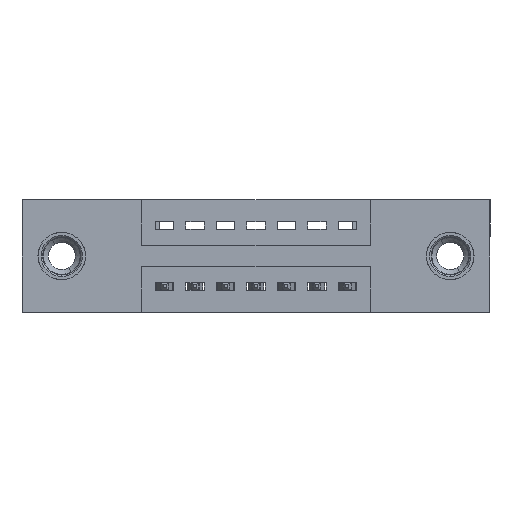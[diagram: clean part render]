
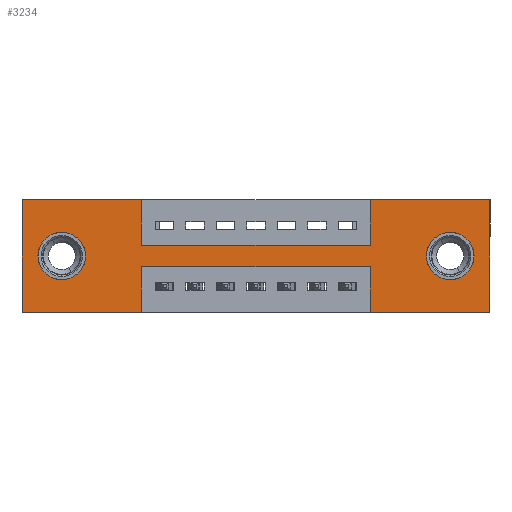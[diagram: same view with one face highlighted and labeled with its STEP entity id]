
A CAD part, front view. The second image highlights one B-rep face of the part: STEP entity #3234.
In plain terms, the highlighted planar face has unit normal (0, -1, 0).
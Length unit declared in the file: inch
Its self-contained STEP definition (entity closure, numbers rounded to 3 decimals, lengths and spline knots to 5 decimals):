
#51 = LINE ( 'NONE', #2546, #246 ) ;
#246 = VECTOR ( 'NONE', #10534, 39.37008 ) ;
#383 = DIRECTION ( 'NONE',  ( 0., -1., 0. ) ) ;
#586 = VERTEX_POINT ( 'NONE', #7537 ) ;
#606 = VERTEX_POINT ( 'NONE', #13101 ) ;
#614 = VERTEX_POINT ( 'NONE', #13140 ) ;
#677 = EDGE_LOOP ( 'NONE', ( #12969, #3364 ) ) ;
#689 = VECTOR ( 'NONE', #7969, 39.37008 ) ;
#757 = ORIENTED_EDGE ( 'NONE', *, *, #4747, .F. ) ;
#789 = EDGE_CURVE ( 'NONE', #6953, #606, #9669, .T. ) ;
#833 = VERTEX_POINT ( 'NONE', #7582 ) ;
#1064 = EDGE_CURVE ( 'NONE', #606, #586, #51, .T. ) ;
#1142 = EDGE_CURVE ( 'NONE', #3409, #6013, #7853, .T. ) ;
#1166 = LINE ( 'NONE', #12140, #6649 ) ;
#1237 = AXIS2_PLACEMENT_3D ( 'NONE', #4250, #4200, #7701 ) ;
#1314 = DIRECTION ( 'NONE',  ( -1., 0., 0. ) ) ;
#1387 = DIRECTION ( 'NONE',  ( 0., 1., 0. ) ) ;
#1470 = LINE ( 'NONE', #12264, #11460 ) ;
#1764 = ORIENTED_EDGE ( 'NONE', *, *, #7753, .F. ) ;
#1964 = CARTESIAN_POINT ( 'NONE',  ( 0., 0., -0.37 ) ) ;
#2014 = ORIENTED_EDGE ( 'NONE', *, *, #13558, .F. ) ;
#2113 = CARTESIAN_POINT ( 'NONE',  ( 0., 0., 0. ) ) ;
#2198 = CARTESIAN_POINT ( 'NONE',  ( 0.13, 0., -0.185 ) ) ;
#2272 = CARTESIAN_POINT ( 'NONE',  ( 0.3925, 0., 0. ) ) ;
#2278 = FACE_BOUND ( 'NONE', #6630, .T. ) ;
#2400 = EDGE_CURVE ( 'NONE', #7085, #12462, #4074, .T. ) ;
#2546 = CARTESIAN_POINT ( 'NONE',  ( 1.1425, 0., -0.37 ) ) ;
#2766 = CARTESIAN_POINT ( 'NONE',  ( 0.3925, 0., -0.22 ) ) ;
#2775 = ORIENTED_EDGE ( 'NONE', *, *, #1142, .T. ) ;
#2956 = CARTESIAN_POINT ( 'NONE',  ( 0.13, 0., -0.263 ) ) ;
#3073 = CARTESIAN_POINT ( 'NONE',  ( 1.535, 0., 0. ) ) ;
#3091 = DIRECTION ( 'NONE',  ( 0., 0., 1. ) ) ;
#3234 = ADVANCED_FACE ( 'NONE', ( #3869, #2278, #10321 ), #11690, .T. ) ;
#3237 = EDGE_LOOP ( 'NONE', ( #12624, #14509, #9939, #12177, #757, #9696, #1764, #8706, #6977, #9450, #2014, #5295 ) ) ;
#3364 = ORIENTED_EDGE ( 'NONE', *, *, #11262, .T. ) ;
#3375 = LINE ( 'NONE', #12848, #5713 ) ;
#3377 = VERTEX_POINT ( 'NONE', #3429 ) ;
#3391 = CARTESIAN_POINT ( 'NONE',  ( 0.3925, 0., -0.15 ) ) ;
#3409 = VERTEX_POINT ( 'NONE', #14288 ) ;
#3429 = CARTESIAN_POINT ( 'NONE',  ( 1.405, 0., -0.263 ) ) ;
#3604 = LINE ( 'NONE', #7805, #10917 ) ;
#3758 = EDGE_CURVE ( 'NONE', #6013, #3409, #10312, .T. ) ;
#3869 = FACE_BOUND ( 'NONE', #677, .T. ) ;
#4074 = LINE ( 'NONE', #5145, #10182 ) ;
#4200 = DIRECTION ( 'NONE',  ( 0., 1., 0. ) ) ;
#4250 = CARTESIAN_POINT ( 'NONE',  ( 1.405, 0., -0.185 ) ) ;
#4520 = LINE ( 'NONE', #13825, #13256 ) ;
#4596 = DIRECTION ( 'NONE',  ( 0., 0., 1. ) ) ;
#4747 = EDGE_CURVE ( 'NONE', #13995, #6953, #8830, .T. ) ;
#5145 = CARTESIAN_POINT ( 'NONE',  ( 0.3925, 0., -0.37 ) ) ;
#5265 = EDGE_CURVE ( 'NONE', #11827, #3377, #8095, .T. ) ;
#5295 = ORIENTED_EDGE ( 'NONE', *, *, #13341, .F. ) ;
#5491 = DIRECTION ( 'NONE',  ( 0., 0., 1. ) ) ;
#5689 = CARTESIAN_POINT ( 'NONE',  ( 0.3925, 0., -0.37 ) ) ;
#5713 = VECTOR ( 'NONE', #6033, 39.37008 ) ;
#6013 = VERTEX_POINT ( 'NONE', #2956 ) ;
#6033 = DIRECTION ( 'NONE',  ( 1., 0., 0. ) ) ;
#6117 = VECTOR ( 'NONE', #3091, 39.37008 ) ;
#6143 = VECTOR ( 'NONE', #7005, 39.37008 ) ;
#6153 = VECTOR ( 'NONE', #9395, 39.37008 ) ;
#6630 = EDGE_LOOP ( 'NONE', ( #2775, #10896 ) ) ;
#6649 = VECTOR ( 'NONE', #10926, 39.37008 ) ;
#6783 = AXIS2_PLACEMENT_3D ( 'NONE', #13932, #383, #10579 ) ;
#6833 = VERTEX_POINT ( 'NONE', #8559 ) ;
#6953 = VERTEX_POINT ( 'NONE', #11120 ) ;
#6977 = ORIENTED_EDGE ( 'NONE', *, *, #14034, .F. ) ;
#7005 = DIRECTION ( 'NONE',  ( 0., 0., -1. ) ) ;
#7085 = VERTEX_POINT ( 'NONE', #2766 ) ;
#7436 = AXIS2_PLACEMENT_3D ( 'NONE', #2198, #9067, #4596 ) ;
#7537 = CARTESIAN_POINT ( 'NONE',  ( 1.1425, 0., -0.22 ) ) ;
#7582 = CARTESIAN_POINT ( 'NONE',  ( 1.1425, 0., 0. ) ) ;
#7633 = DIRECTION ( 'NONE',  ( -1., 0., 0. ) ) ;
#7701 = DIRECTION ( 'NONE',  ( 0., 0., -1. ) ) ;
#7753 = EDGE_CURVE ( 'NONE', #11505, #833, #1470, .T. ) ;
#7805 = CARTESIAN_POINT ( 'NONE',  ( 0.3925, 0., 0. ) ) ;
#7853 = CIRCLE ( 'NONE', #7436, 0.078 ) ;
#7969 = DIRECTION ( 'NONE',  ( 1., 0., 0. ) ) ;
#8095 = CIRCLE ( 'NONE', #1237, 0.078 ) ;
#8124 = CARTESIAN_POINT ( 'NONE',  ( 0., 0., 0. ) ) ;
#8167 = AXIS2_PLACEMENT_3D ( 'NONE', #11703, #1387, #11555 ) ;
#8315 = CARTESIAN_POINT ( 'NONE',  ( 1.535, 0., 0. ) ) ;
#8559 = CARTESIAN_POINT ( 'NONE',  ( 0.3925, 0., -0.15 ) ) ;
#8629 = DIRECTION ( 'NONE',  ( 0., 0., -1. ) ) ;
#8706 = ORIENTED_EDGE ( 'NONE', *, *, #11588, .F. ) ;
#8830 = LINE ( 'NONE', #8315, #6143 ) ;
#8832 = CARTESIAN_POINT ( 'NONE',  ( 1.405, 0., -0.107 ) ) ;
#8913 = DIRECTION ( 'NONE',  ( 0., 0., -1. ) ) ;
#8928 = CARTESIAN_POINT ( 'NONE',  ( 1.405, 0., -0.185 ) ) ;
#8985 = EDGE_CURVE ( 'NONE', #614, #12992, #3375, .T. ) ;
#9067 = DIRECTION ( 'NONE',  ( 0., 1., 0. ) ) ;
#9395 = DIRECTION ( 'NONE',  ( 1., 0., 0. ) ) ;
#9415 = CARTESIAN_POINT ( 'NONE',  ( 1.1425, 0., -0.15 ) ) ;
#9450 = ORIENTED_EDGE ( 'NONE', *, *, #8985, .F. ) ;
#9669 = LINE ( 'NONE', #1964, #10912 ) ;
#9696 = ORIENTED_EDGE ( 'NONE', *, *, #10755, .F. ) ;
#9939 = ORIENTED_EDGE ( 'NONE', *, *, #1064, .F. ) ;
#10182 = VECTOR ( 'NONE', #8629, 39.37008 ) ;
#10250 = DIRECTION ( 'NONE',  ( 0., 0., -1. ) ) ;
#10312 = CIRCLE ( 'NONE', #8167, 0.078 ) ;
#10321 = FACE_OUTER_BOUND ( 'NONE', #3237, .T. ) ;
#10436 = VERTEX_POINT ( 'NONE', #11675 ) ;
#10534 = DIRECTION ( 'NONE',  ( 0., 0., 1. ) ) ;
#10579 = DIRECTION ( 'NONE',  ( 0., 0., -1. ) ) ;
#10755 = EDGE_CURVE ( 'NONE', #833, #13995, #12820, .T. ) ;
#10896 = ORIENTED_EDGE ( 'NONE', *, *, #3758, .T. ) ;
#10912 = VECTOR ( 'NONE', #7633, 39.37008 ) ;
#10917 = VECTOR ( 'NONE', #8913, 39.37008 ) ;
#10926 = DIRECTION ( 'NONE',  ( -1., 0., 0. ) ) ;
#10986 = LINE ( 'NONE', #3391, #6153 ) ;
#11120 = CARTESIAN_POINT ( 'NONE',  ( 1.535, 0., -0.37 ) ) ;
#11262 = EDGE_CURVE ( 'NONE', #3377, #11827, #11728, .T. ) ;
#11435 = DIRECTION ( 'NONE',  ( 0., 1., 0. ) ) ;
#11460 = VECTOR ( 'NONE', #5491, 39.37008 ) ;
#11505 = VERTEX_POINT ( 'NONE', #9415 ) ;
#11555 = DIRECTION ( 'NONE',  ( 0., 0., 1. ) ) ;
#11588 = EDGE_CURVE ( 'NONE', #6833, #11505, #10986, .T. ) ;
#11675 = CARTESIAN_POINT ( 'NONE',  ( 0., 0., -0.37 ) ) ;
#11690 = PLANE ( 'NONE',  #6783 ) ;
#11703 = CARTESIAN_POINT ( 'NONE',  ( 0.13, 0., -0.185 ) ) ;
#11728 = CIRCLE ( 'NONE', #12155, 0.078 ) ;
#11827 = VERTEX_POINT ( 'NONE', #8832 ) ;
#12140 = CARTESIAN_POINT ( 'NONE',  ( 0., 0., -0.37 ) ) ;
#12155 = AXIS2_PLACEMENT_3D ( 'NONE', #8928, #11435, #10250 ) ;
#12177 = ORIENTED_EDGE ( 'NONE', *, *, #789, .F. ) ;
#12264 = CARTESIAN_POINT ( 'NONE',  ( 1.1425, 0., 0. ) ) ;
#12462 = VERTEX_POINT ( 'NONE', #5689 ) ;
#12624 = ORIENTED_EDGE ( 'NONE', *, *, #2400, .F. ) ;
#12820 = LINE ( 'NONE', #8124, #689 ) ;
#12848 = CARTESIAN_POINT ( 'NONE',  ( 0., 0., 0. ) ) ;
#12969 = ORIENTED_EDGE ( 'NONE', *, *, #5265, .T. ) ;
#12992 = VERTEX_POINT ( 'NONE', #2272 ) ;
#13101 = CARTESIAN_POINT ( 'NONE',  ( 1.1425, 0., -0.37 ) ) ;
#13140 = CARTESIAN_POINT ( 'NONE',  ( 0., 0., 0. ) ) ;
#13256 = VECTOR ( 'NONE', #1314, 39.37008 ) ;
#13341 = EDGE_CURVE ( 'NONE', #12462, #10436, #1166, .T. ) ;
#13441 = LINE ( 'NONE', #2113, #6117 ) ;
#13558 = EDGE_CURVE ( 'NONE', #10436, #614, #13441, .T. ) ;
#13825 = CARTESIAN_POINT ( 'NONE',  ( 0.3925, 0., -0.22 ) ) ;
#13932 = CARTESIAN_POINT ( 'NONE',  ( 0., 0., -0.37 ) ) ;
#13995 = VERTEX_POINT ( 'NONE', #3073 ) ;
#14034 = EDGE_CURVE ( 'NONE', #12992, #6833, #3604, .T. ) ;
#14156 = EDGE_CURVE ( 'NONE', #586, #7085, #4520, .T. ) ;
#14288 = CARTESIAN_POINT ( 'NONE',  ( 0.13, 0., -0.107 ) ) ;
#14509 = ORIENTED_EDGE ( 'NONE', *, *, #14156, .F. ) ;
